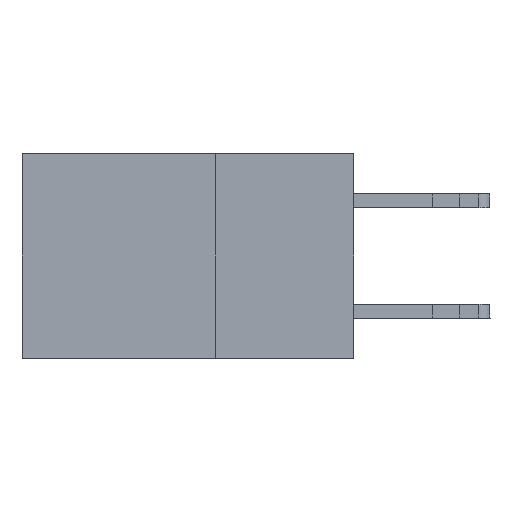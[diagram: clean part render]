
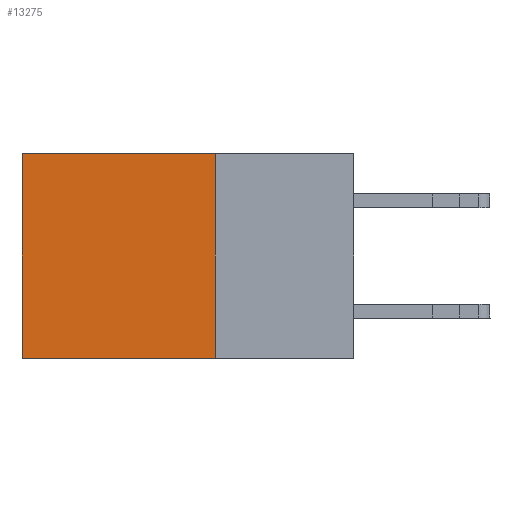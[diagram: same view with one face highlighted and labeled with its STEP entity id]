
A CAD part, left-side view. The second image highlights one B-rep face of the part: STEP entity #13275.
In plain terms, the highlighted planar face has unit normal (-1, 0, 0).
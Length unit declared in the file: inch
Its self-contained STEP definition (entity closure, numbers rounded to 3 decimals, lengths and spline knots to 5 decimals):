
#257 = DIRECTION ( 'NONE',  ( 0., 0., -1. ) ) ;
#563 = EDGE_CURVE ( 'NONE', #11333, #15581, #1908, .T. ) ;
#661 = CARTESIAN_POINT ( 'NONE',  ( 0.2875, 0.25, 0. ) ) ;
#747 = ORIENTED_EDGE ( 'NONE', *, *, #563, .F. ) ;
#1490 = EDGE_CURVE ( 'NONE', #11398, #2570, #14357, .T. ) ;
#1908 = LINE ( 'NONE', #4521, #7700 ) ;
#1959 = PLANE ( 'NONE',  #7661 ) ;
#2080 = EDGE_LOOP ( 'NONE', ( #12330, #4420, #747, #15223 ) ) ;
#2570 = VERTEX_POINT ( 'NONE', #5596 ) ;
#2910 = VECTOR ( 'NONE', #7577, 39.37008 ) ;
#3379 = EDGE_CURVE ( 'NONE', #11333, #11398, #9090, .T. ) ;
#4276 = DIRECTION ( 'NONE',  ( 0., 1., 0. ) ) ;
#4420 = ORIENTED_EDGE ( 'NONE', *, *, #16346, .F. ) ;
#4521 = CARTESIAN_POINT ( 'NONE',  ( 0.2875, 0.25, 0. ) ) ;
#4615 = DIRECTION ( 'NONE',  ( 0., 0., -1. ) ) ;
#5596 = CARTESIAN_POINT ( 'NONE',  ( 0.2875, 0.6, -0.37 ) ) ;
#5796 = VECTOR ( 'NONE', #4276, 39.37008 ) ;
#6165 = CARTESIAN_POINT ( 'NONE',  ( 0.2875, 0.6, 0. ) ) ;
#6432 = CARTESIAN_POINT ( 'NONE',  ( 0.2875, 0.6, 0. ) ) ;
#7577 = DIRECTION ( 'NONE',  ( 0., 1., 0. ) ) ;
#7600 = CARTESIAN_POINT ( 'NONE',  ( 0.2875, 0.25, 0. ) ) ;
#7661 = AXIS2_PLACEMENT_3D ( 'NONE', #661, #12327, #4615 ) ;
#7671 = VECTOR ( 'NONE', #257, 39.37008 ) ;
#7700 = VECTOR ( 'NONE', #14971, 39.37008 ) ;
#8554 = FACE_OUTER_BOUND ( 'NONE', #2080, .T. ) ;
#9090 = LINE ( 'NONE', #12129, #2910 ) ;
#11333 = VERTEX_POINT ( 'NONE', #7600 ) ;
#11398 = VERTEX_POINT ( 'NONE', #6432 ) ;
#11827 = CARTESIAN_POINT ( 'NONE',  ( 0.2875, 0.25, -0.37 ) ) ;
#12019 = CARTESIAN_POINT ( 'NONE',  ( 0.2875, 0.25, -0.37 ) ) ;
#12129 = CARTESIAN_POINT ( 'NONE',  ( 0.2875, 0.25, 0. ) ) ;
#12327 = DIRECTION ( 'NONE',  ( 1., 0., 0. ) ) ;
#12330 = ORIENTED_EDGE ( 'NONE', *, *, #1490, .T. ) ;
#13275 = ADVANCED_FACE ( 'NONE', ( #8554 ), #1959, .F. ) ;
#14357 = LINE ( 'NONE', #6165, #7671 ) ;
#14971 = DIRECTION ( 'NONE',  ( 0., 0., -1. ) ) ;
#15223 = ORIENTED_EDGE ( 'NONE', *, *, #3379, .T. ) ;
#15511 = LINE ( 'NONE', #12019, #5796 ) ;
#15581 = VERTEX_POINT ( 'NONE', #11827 ) ;
#16346 = EDGE_CURVE ( 'NONE', #15581, #2570, #15511, .T. ) ;
